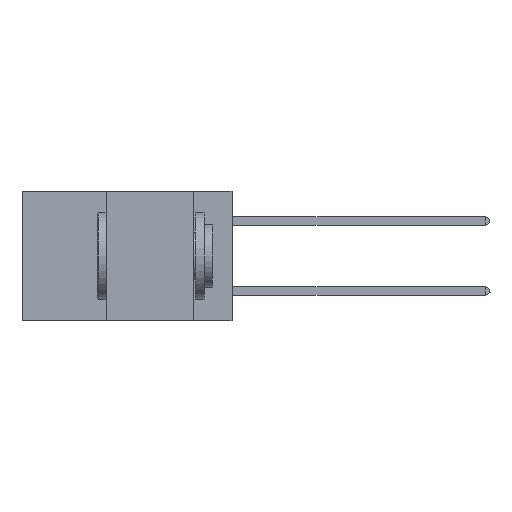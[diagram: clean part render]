
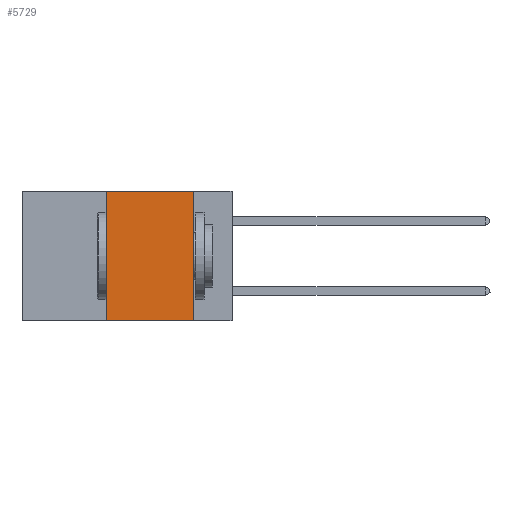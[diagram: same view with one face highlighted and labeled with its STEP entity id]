
A CAD part, left-side view. The second image highlights one B-rep face of the part: STEP entity #5729.
In plain terms, the highlighted planar face has unit normal (-1, 0, 0).
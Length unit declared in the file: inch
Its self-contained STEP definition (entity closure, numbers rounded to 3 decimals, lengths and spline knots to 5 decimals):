
#2045 = VECTOR ( 'NONE', #14151, 39.37008 ) ;
#2329 = VERTEX_POINT ( 'NONE', #6707 ) ;
#3081 = AXIS2_PLACEMENT_3D ( 'NONE', #12934, #15775, #17119 ) ;
#4192 = EDGE_CURVE ( 'NONE', #8302, #2329, #12782, .T. ) ;
#4711 = CARTESIAN_POINT ( 'NONE',  ( 0., 0.11, 0. ) ) ;
#4957 = CARTESIAN_POINT ( 'NONE',  ( 0., 0.36, 0. ) ) ;
#4974 = PLANE ( 'NONE',  #3081 ) ;
#5356 = ORIENTED_EDGE ( 'NONE', *, *, #7276, .F. ) ;
#5729 = ADVANCED_FACE ( 'NONE', ( #12093 ), #4974, .F. ) ;
#6707 = CARTESIAN_POINT ( 'NONE',  ( 0., 0.11, 0. ) ) ;
#6754 = DIRECTION ( 'NONE',  ( 0., -1., 0. ) ) ;
#7276 = EDGE_CURVE ( 'NONE', #12199, #8302, #9917, .T. ) ;
#8039 = LINE ( 'NONE', #10633, #11225 ) ;
#8287 = EDGE_CURVE ( 'NONE', #12199, #9507, #8039, .T. ) ;
#8302 = VERTEX_POINT ( 'NONE', #4957 ) ;
#9015 = LINE ( 'NONE', #4711, #2045 ) ;
#9154 = DIRECTION ( 'NONE',  ( 0., 0., 1. ) ) ;
#9236 = CARTESIAN_POINT ( 'NONE',  ( 0., 0.6, 0. ) ) ;
#9461 = ORIENTED_EDGE ( 'NONE', *, *, #14971, .F. ) ;
#9507 = VERTEX_POINT ( 'NONE', #12295 ) ;
#9917 = LINE ( 'NONE', #16118, #10153 ) ;
#10153 = VECTOR ( 'NONE', #9154, 39.37008 ) ;
#10633 = CARTESIAN_POINT ( 'NONE',  ( 0., 0.6, -0.37 ) ) ;
#11225 = VECTOR ( 'NONE', #14565, 39.37008 ) ;
#12093 = FACE_OUTER_BOUND ( 'NONE', #13530, .T. ) ;
#12199 = VERTEX_POINT ( 'NONE', #12916 ) ;
#12295 = CARTESIAN_POINT ( 'NONE',  ( 0., 0.11, -0.37 ) ) ;
#12615 = ORIENTED_EDGE ( 'NONE', *, *, #8287, .T. ) ;
#12764 = VECTOR ( 'NONE', #6754, 39.37008 ) ;
#12782 = LINE ( 'NONE', #9236, #12764 ) ;
#12916 = CARTESIAN_POINT ( 'NONE',  ( 0., 0.36, -0.37 ) ) ;
#12934 = CARTESIAN_POINT ( 'NONE',  ( 0., 0.6, 0. ) ) ;
#13530 = EDGE_LOOP ( 'NONE', ( #9461, #14028, #5356, #12615 ) ) ;
#14028 = ORIENTED_EDGE ( 'NONE', *, *, #4192, .F. ) ;
#14151 = DIRECTION ( 'NONE',  ( 0., 0., -1. ) ) ;
#14565 = DIRECTION ( 'NONE',  ( 0., -1., 0. ) ) ;
#14971 = EDGE_CURVE ( 'NONE', #2329, #9507, #9015, .T. ) ;
#15775 = DIRECTION ( 'NONE',  ( 1., 0., 0. ) ) ;
#16118 = CARTESIAN_POINT ( 'NONE',  ( 0., 0.36, 0. ) ) ;
#17119 = DIRECTION ( 'NONE',  ( 0., 0., -1. ) ) ;
